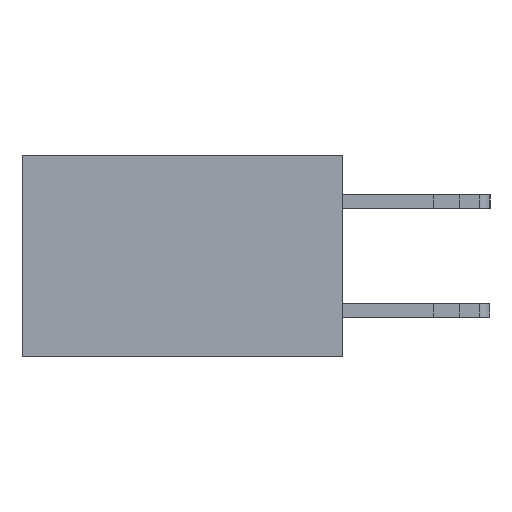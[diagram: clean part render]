
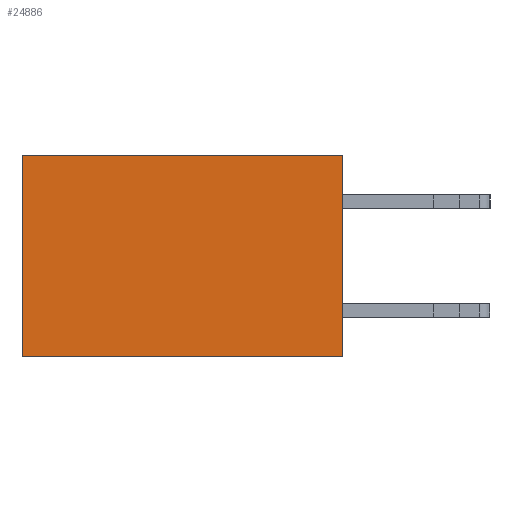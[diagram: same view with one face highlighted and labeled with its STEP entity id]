
A CAD part, left-side view. The second image highlights one B-rep face of the part: STEP entity #24886.
In plain terms, the highlighted planar face has unit normal (-1, 0, 0).
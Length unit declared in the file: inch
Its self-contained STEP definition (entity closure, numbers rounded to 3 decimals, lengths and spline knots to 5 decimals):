
#52 = VERTEX_POINT ( 'NONE', #19142 ) ;
#290 = EDGE_LOOP ( 'NONE', ( #1002, #2849, #12396, #16136 ) ) ;
#483 = VERTEX_POINT ( 'NONE', #4984 ) ;
#533 = DIRECTION ( 'NONE',  ( 0., 0., -1. ) ) ;
#681 = CARTESIAN_POINT ( 'NONE',  ( 0.277, 0.59, -0.37 ) ) ;
#1002 = ORIENTED_EDGE ( 'NONE', *, *, #10811, .T. ) ;
#2234 = DIRECTION ( 'NONE',  ( 0., 0., -1. ) ) ;
#2329 = CARTESIAN_POINT ( 'NONE',  ( 0.277, 0., 0. ) ) ;
#2849 = ORIENTED_EDGE ( 'NONE', *, *, #11804, .F. ) ;
#4984 = CARTESIAN_POINT ( 'NONE',  ( 0.277, 0.59, 0. ) ) ;
#6942 = PLANE ( 'NONE',  #25771 ) ;
#7763 = CARTESIAN_POINT ( 'NONE',  ( 0.277, 0., -0.37 ) ) ;
#8671 = LINE ( 'NONE', #7763, #20592 ) ;
#9660 = EDGE_CURVE ( 'NONE', #27718, #52, #12159, .T. ) ;
#10811 = EDGE_CURVE ( 'NONE', #483, #23696, #23569, .T. ) ;
#10957 = VECTOR ( 'NONE', #533, 39.37008 ) ;
#11804 = EDGE_CURVE ( 'NONE', #52, #23696, #8671, .T. ) ;
#12159 = LINE ( 'NONE', #26945, #18484 ) ;
#12372 = CARTESIAN_POINT ( 'NONE',  ( 0.277, 0., 0. ) ) ;
#12396 = ORIENTED_EDGE ( 'NONE', *, *, #9660, .F. ) ;
#15120 = EDGE_CURVE ( 'NONE', #27718, #483, #18890, .T. ) ;
#16136 = ORIENTED_EDGE ( 'NONE', *, *, #15120, .T. ) ;
#16526 = DIRECTION ( 'NONE',  ( 1., 0., 0. ) ) ;
#18143 = VECTOR ( 'NONE', #26010, 39.37008 ) ;
#18484 = VECTOR ( 'NONE', #27247, 39.37008 ) ;
#18890 = LINE ( 'NONE', #2329, #18143 ) ;
#19142 = CARTESIAN_POINT ( 'NONE',  ( 0.277, 0., -0.37 ) ) ;
#19638 = DIRECTION ( 'NONE',  ( 0., 1., 0. ) ) ;
#20592 = VECTOR ( 'NONE', #19638, 39.37008 ) ;
#23569 = LINE ( 'NONE', #681, #10957 ) ;
#23696 = VERTEX_POINT ( 'NONE', #24222 ) ;
#24222 = CARTESIAN_POINT ( 'NONE',  ( 0.277, 0.59, -0.37 ) ) ;
#24886 = ADVANCED_FACE ( 'NONE', ( #28848 ), #6942, .F. ) ;
#25771 = AXIS2_PLACEMENT_3D ( 'NONE', #30557, #16526, #2234 ) ;
#26010 = DIRECTION ( 'NONE',  ( 0., 1., 0. ) ) ;
#26945 = CARTESIAN_POINT ( 'NONE',  ( 0.277, 0., -0.37 ) ) ;
#27247 = DIRECTION ( 'NONE',  ( 0., 0., -1. ) ) ;
#27718 = VERTEX_POINT ( 'NONE', #12372 ) ;
#28848 = FACE_OUTER_BOUND ( 'NONE', #290, .T. ) ;
#30557 = CARTESIAN_POINT ( 'NONE',  ( 0.277, 0., -0.37 ) ) ;
